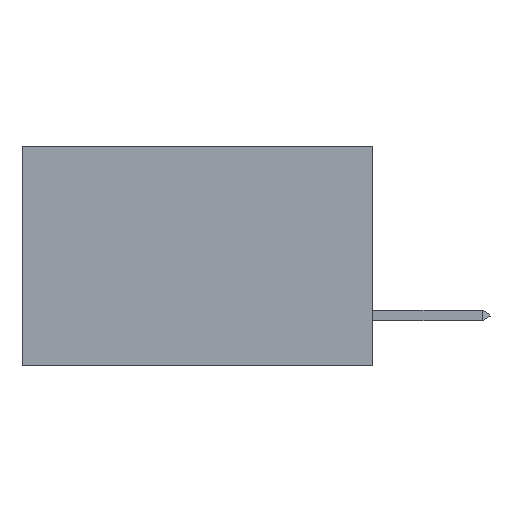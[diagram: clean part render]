
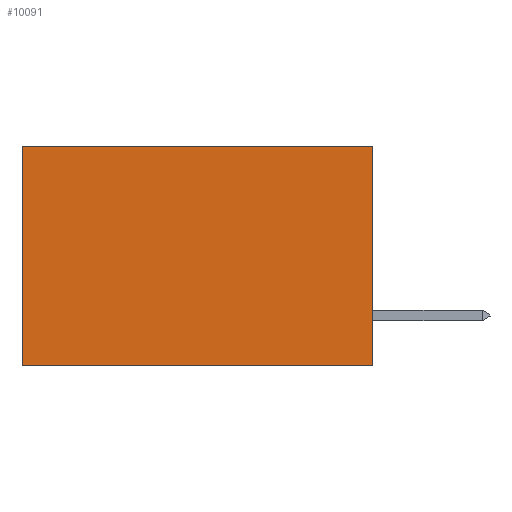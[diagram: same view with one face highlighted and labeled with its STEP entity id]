
A CAD part, left-side view. The second image highlights one B-rep face of the part: STEP entity #10091.
In plain terms, the highlighted planar face has unit normal (-1, 0, 0).
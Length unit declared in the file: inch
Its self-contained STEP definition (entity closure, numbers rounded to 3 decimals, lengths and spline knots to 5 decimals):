
#153 = ORIENTED_EDGE ( 'NONE', *, *, #2859, .T. ) ;
#171 = EDGE_CURVE ( 'NONE', #2167, #7228, #7606, .T. ) ;
#638 = DIRECTION ( 'NONE',  ( 0., 0., -1. ) ) ;
#820 = LINE ( 'NONE', #3505, #9008 ) ;
#1318 = LINE ( 'NONE', #11863, #10132 ) ;
#2167 = VERTEX_POINT ( 'NONE', #2756 ) ;
#2283 = CARTESIAN_POINT ( 'NONE',  ( 0.277, 0.59, -0.37 ) ) ;
#2756 = CARTESIAN_POINT ( 'NONE',  ( 0.277, 0.59, 0. ) ) ;
#2859 = EDGE_CURVE ( 'NONE', #9774, #2167, #1318, .T. ) ;
#3065 = ORIENTED_EDGE ( 'NONE', *, *, #7009, .F. ) ;
#3222 = ORIENTED_EDGE ( 'NONE', *, *, #171, .T. ) ;
#3505 = CARTESIAN_POINT ( 'NONE',  ( 0.277, 0., -0.37 ) ) ;
#3581 = DIRECTION ( 'NONE',  ( 0., 1., 0. ) ) ;
#3942 = EDGE_LOOP ( 'NONE', ( #3222, #3065, #7830, #153 ) ) ;
#4238 = CARTESIAN_POINT ( 'NONE',  ( 0.277, 0., -0.37 ) ) ;
#4926 = AXIS2_PLACEMENT_3D ( 'NONE', #4238, #7687, #638 ) ;
#5291 = DIRECTION ( 'NONE',  ( 0., 1., 0. ) ) ;
#5700 = VECTOR ( 'NONE', #12832, 39.37008 ) ;
#5776 = EDGE_CURVE ( 'NONE', #9774, #6465, #8349, .T. ) ;
#6465 = VERTEX_POINT ( 'NONE', #7061 ) ;
#7009 = EDGE_CURVE ( 'NONE', #6465, #7228, #820, .T. ) ;
#7061 = CARTESIAN_POINT ( 'NONE',  ( 0.277, 0., -0.37 ) ) ;
#7228 = VERTEX_POINT ( 'NONE', #2283 ) ;
#7606 = LINE ( 'NONE', #11866, #13340 ) ;
#7687 = DIRECTION ( 'NONE',  ( 1., 0., 0. ) ) ;
#7830 = ORIENTED_EDGE ( 'NONE', *, *, #5776, .F. ) ;
#8349 = LINE ( 'NONE', #12952, #5700 ) ;
#9008 = VECTOR ( 'NONE', #3581, 39.37008 ) ;
#9774 = VERTEX_POINT ( 'NONE', #10466 ) ;
#10091 = ADVANCED_FACE ( 'NONE', ( #14552 ), #14175, .F. ) ;
#10132 = VECTOR ( 'NONE', #5291, 39.37008 ) ;
#10466 = CARTESIAN_POINT ( 'NONE',  ( 0.277, 0., 0. ) ) ;
#11850 = DIRECTION ( 'NONE',  ( 0., 0., -1. ) ) ;
#11863 = CARTESIAN_POINT ( 'NONE',  ( 0.277, 0., 0. ) ) ;
#11866 = CARTESIAN_POINT ( 'NONE',  ( 0.277, 0.59, -0.37 ) ) ;
#12832 = DIRECTION ( 'NONE',  ( 0., 0., -1. ) ) ;
#12952 = CARTESIAN_POINT ( 'NONE',  ( 0.277, 0., -0.37 ) ) ;
#13340 = VECTOR ( 'NONE', #11850, 39.37008 ) ;
#14175 = PLANE ( 'NONE',  #4926 ) ;
#14552 = FACE_OUTER_BOUND ( 'NONE', #3942, .T. ) ;
